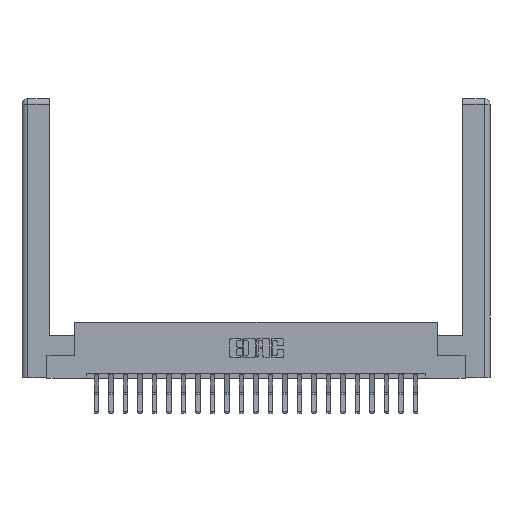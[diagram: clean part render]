
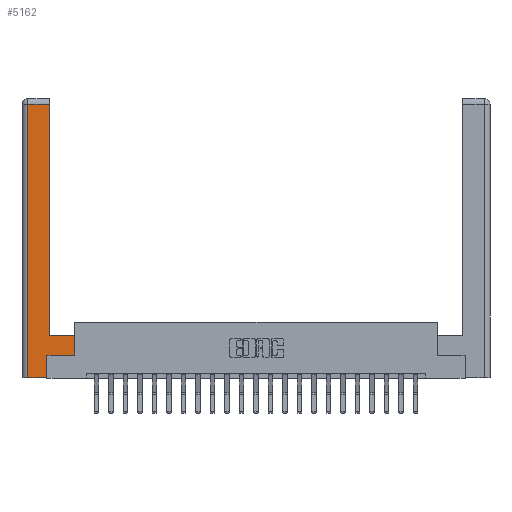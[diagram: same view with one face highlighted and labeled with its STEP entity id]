
A CAD part, top view. The second image highlights one B-rep face of the part: STEP entity #5162.
In plain terms, the highlighted planar face has unit normal (0, 0, 1).
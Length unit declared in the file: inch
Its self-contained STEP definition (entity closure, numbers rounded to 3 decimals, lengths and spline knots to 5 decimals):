
#162 = DIRECTION ( 'NONE',  ( -1., 0., 0. ) ) ;
#1028 = CARTESIAN_POINT ( 'NONE',  ( 0.0615, 0., 0. ) ) ;
#1054 = ORIENTED_EDGE ( 'NONE', *, *, #10216, .T. ) ;
#1522 = LINE ( 'NONE', #19301, #5111 ) ;
#1704 = VERTEX_POINT ( 'NONE', #15310 ) ;
#1927 = CARTESIAN_POINT ( 'NONE',  ( 0.265, 0., 0. ) ) ;
#2042 = EDGE_CURVE ( 'NONE', #10555, #6364, #6094, .T. ) ;
#2119 = CARTESIAN_POINT ( 'NONE',  ( 0.0615, 2.94, 0. ) ) ;
#2446 = VECTOR ( 'NONE', #162, 39.37008 ) ;
#2515 = ORIENTED_EDGE ( 'NONE', *, *, #19124, .T. ) ;
#3239 = VECTOR ( 'NONE', #13429, 39.37008 ) ;
#4108 = CARTESIAN_POINT ( 'NONE',  ( 0.0615, 2.94, 0. ) ) ;
#4457 = CARTESIAN_POINT ( 'NONE',  ( 0.265, 0.245, 0. ) ) ;
#5111 = VECTOR ( 'NONE', #8628, 39.37008 ) ;
#5162 = ADVANCED_FACE ( 'NONE', ( #9842 ), #12524, .F. ) ;
#5468 = EDGE_CURVE ( 'NONE', #10997, #12688, #5924, .T. ) ;
#5626 = LINE ( 'NONE', #4457, #6721 ) ;
#5924 = LINE ( 'NONE', #7040, #18738 ) ;
#6094 = LINE ( 'NONE', #1927, #6382 ) ;
#6364 = VERTEX_POINT ( 'NONE', #14718 ) ;
#6382 = VECTOR ( 'NONE', #7426, 39.37008 ) ;
#6721 = VECTOR ( 'NONE', #15032, 39.37008 ) ;
#7040 = CARTESIAN_POINT ( 'NONE',  ( 0.295, 3., 0. ) ) ;
#7426 = DIRECTION ( 'NONE',  ( 1., 0., 0. ) ) ;
#7575 = CARTESIAN_POINT ( 'NONE',  ( 0.565, 0.45, 0. ) ) ;
#7868 = CARTESIAN_POINT ( 'NONE',  ( 0.0615, 0., 0. ) ) ;
#7986 = LINE ( 'NONE', #4108, #21343 ) ;
#8294 = VECTOR ( 'NONE', #19057, 39.37008 ) ;
#8628 = DIRECTION ( 'NONE',  ( 1., 0., 0. ) ) ;
#9169 = CARTESIAN_POINT ( 'NONE',  ( 0.295, 0.45, 0. ) ) ;
#9233 = EDGE_CURVE ( 'NONE', #21199, #10555, #17168, .T. ) ;
#9340 = EDGE_CURVE ( 'NONE', #12688, #21199, #7986, .T. ) ;
#9657 = LINE ( 'NONE', #9169, #2446 ) ;
#9842 = FACE_OUTER_BOUND ( 'NONE', #12447, .T. ) ;
#9964 = LINE ( 'NONE', #18836, #8294 ) ;
#10216 = EDGE_CURVE ( 'NONE', #17507, #1704, #1522, .T. ) ;
#10491 = EDGE_CURVE ( 'NONE', #6364, #17507, #5626, .T. ) ;
#10555 = VERTEX_POINT ( 'NONE', #7868 ) ;
#10997 = VERTEX_POINT ( 'NONE', #18068 ) ;
#11013 = ORIENTED_EDGE ( 'NONE', *, *, #9233, .T. ) ;
#12447 = EDGE_LOOP ( 'NONE', ( #16101, #14376, #11013, #14868, #22691, #1054, #2515, #18333 ) ) ;
#12524 = PLANE ( 'NONE',  #18454 ) ;
#12688 = VERTEX_POINT ( 'NONE', #13980 ) ;
#13294 = EDGE_CURVE ( 'NONE', #17858, #10997, #9657, .T. ) ;
#13429 = DIRECTION ( 'NONE',  ( 0., -1., 0. ) ) ;
#13980 = CARTESIAN_POINT ( 'NONE',  ( 0.295, 2.94, 0. ) ) ;
#14376 = ORIENTED_EDGE ( 'NONE', *, *, #9340, .T. ) ;
#14718 = CARTESIAN_POINT ( 'NONE',  ( 0.265, 0., 0. ) ) ;
#14868 = ORIENTED_EDGE ( 'NONE', *, *, #2042, .T. ) ;
#15032 = DIRECTION ( 'NONE',  ( 0., 1., 0. ) ) ;
#15310 = CARTESIAN_POINT ( 'NONE',  ( 0.565, 0.245, 0. ) ) ;
#16101 = ORIENTED_EDGE ( 'NONE', *, *, #5468, .T. ) ;
#16692 = DIRECTION ( 'NONE',  ( -1., 0., 0. ) ) ;
#17168 = LINE ( 'NONE', #1028, #3239 ) ;
#17507 = VERTEX_POINT ( 'NONE', #20466 ) ;
#17858 = VERTEX_POINT ( 'NONE', #7575 ) ;
#17933 = DIRECTION ( 'NONE',  ( 0., 0., -1. ) ) ;
#18068 = CARTESIAN_POINT ( 'NONE',  ( 0.295, 0.45, 0. ) ) ;
#18333 = ORIENTED_EDGE ( 'NONE', *, *, #13294, .T. ) ;
#18454 = AXIS2_PLACEMENT_3D ( 'NONE', #21741, #17933, #21656 ) ;
#18738 = VECTOR ( 'NONE', #21045, 39.37008 ) ;
#18836 = CARTESIAN_POINT ( 'NONE',  ( 0.565, 0.45, 0. ) ) ;
#19057 = DIRECTION ( 'NONE',  ( 0., 1., 0. ) ) ;
#19124 = EDGE_CURVE ( 'NONE', #1704, #17858, #9964, .T. ) ;
#19301 = CARTESIAN_POINT ( 'NONE',  ( 0.565, 0.245, 0. ) ) ;
#20466 = CARTESIAN_POINT ( 'NONE',  ( 0.265, 0.245, 0. ) ) ;
#21045 = DIRECTION ( 'NONE',  ( 0., 1., 0. ) ) ;
#21199 = VERTEX_POINT ( 'NONE', #2119 ) ;
#21343 = VECTOR ( 'NONE', #16692, 39.37008 ) ;
#21656 = DIRECTION ( 'NONE',  ( -1., 0., 0. ) ) ;
#21741 = CARTESIAN_POINT ( 'NONE',  ( 0., 0., 0. ) ) ;
#22691 = ORIENTED_EDGE ( 'NONE', *, *, #10491, .T. ) ;
